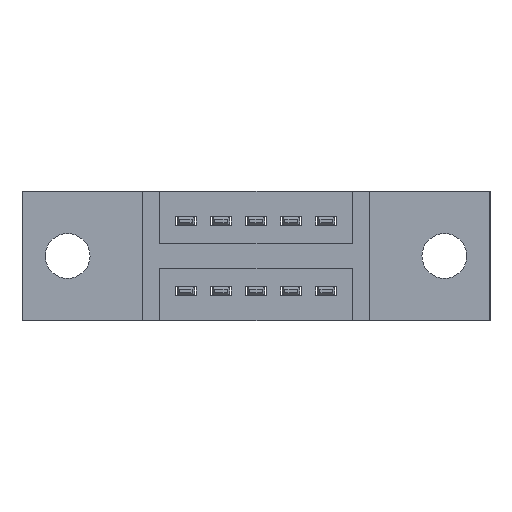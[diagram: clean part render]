
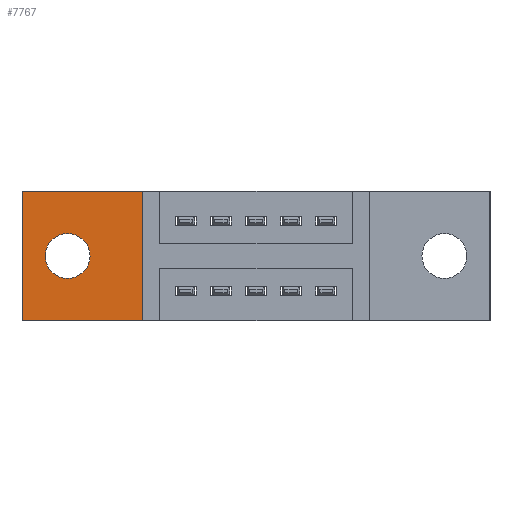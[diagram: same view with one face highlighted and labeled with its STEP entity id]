
A CAD part, front view. The second image highlights one B-rep face of the part: STEP entity #7767.
In plain terms, the highlighted planar face has unit normal (0, -1, 0).
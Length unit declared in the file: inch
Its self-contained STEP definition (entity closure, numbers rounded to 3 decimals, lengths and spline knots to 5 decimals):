
#136 = EDGE_LOOP ( 'NONE', ( #8341, #6078, #2822, #6022 ) ) ;
#354 = FACE_BOUND ( 'NONE', #4602, .T. ) ;
#615 = CARTESIAN_POINT ( 'NONE',  ( 0.3425, 0.17, 0. ) ) ;
#656 = VERTEX_POINT ( 'NONE', #5171 ) ;
#828 = DIRECTION ( 'NONE',  ( 0., 0., 1. ) ) ;
#831 = VERTEX_POINT ( 'NONE', #1865 ) ;
#839 = FACE_OUTER_BOUND ( 'NONE', #136, .T. ) ;
#1080 = CARTESIAN_POINT ( 'NONE',  ( 0., 0.17, -0.37 ) ) ;
#1251 = CARTESIAN_POINT ( 'NONE',  ( 0., 0.17, 0. ) ) ;
#1278 = DIRECTION ( 'NONE',  ( 0., 0., -1. ) ) ;
#1450 = CARTESIAN_POINT ( 'NONE',  ( 0.13, 0.17, -0.185 ) ) ;
#1543 = DIRECTION ( 'NONE',  ( 0., -1., 0. ) ) ;
#1711 = CARTESIAN_POINT ( 'NONE',  ( 0., 0.17, -0.37 ) ) ;
#1865 = CARTESIAN_POINT ( 'NONE',  ( 0.13, 0.17, -0.121 ) ) ;
#1981 = CIRCLE ( 'NONE', #6103, 0.064 ) ;
#2098 = VECTOR ( 'NONE', #1278, 39.37008 ) ;
#2188 = CARTESIAN_POINT ( 'NONE',  ( 0.13, 0.17, -0.249 ) ) ;
#2214 = VERTEX_POINT ( 'NONE', #5111 ) ;
#2232 = EDGE_CURVE ( 'NONE', #656, #2904, #4219, .T. ) ;
#2291 = VECTOR ( 'NONE', #828, 39.37008 ) ;
#2439 = LINE ( 'NONE', #1711, #7256 ) ;
#2822 = ORIENTED_EDGE ( 'NONE', *, *, #2232, .T. ) ;
#2904 = VERTEX_POINT ( 'NONE', #3269 ) ;
#3015 = CIRCLE ( 'NONE', #4152, 0.064 ) ;
#3106 = LINE ( 'NONE', #3818, #4953 ) ;
#3231 = DIRECTION ( 'NONE',  ( 0., -1., 0. ) ) ;
#3252 = VERTEX_POINT ( 'NONE', #2188 ) ;
#3269 = CARTESIAN_POINT ( 'NONE',  ( 0.3425, 0.17, 0. ) ) ;
#3818 = CARTESIAN_POINT ( 'NONE',  ( 0., 0.17, 0. ) ) ;
#4000 = LINE ( 'NONE', #1251, #2098 ) ;
#4152 = AXIS2_PLACEMENT_3D ( 'NONE', #1450, #1543, #6845 ) ;
#4219 = LINE ( 'NONE', #615, #2291 ) ;
#4441 = DIRECTION ( 'NONE',  ( -1., 0., 0. ) ) ;
#4602 = EDGE_LOOP ( 'NONE', ( #8755, #7608 ) ) ;
#4606 = EDGE_CURVE ( 'NONE', #3252, #831, #3015, .T. ) ;
#4778 = VERTEX_POINT ( 'NONE', #7077 ) ;
#4953 = VECTOR ( 'NONE', #4441, 39.37008 ) ;
#5095 = EDGE_CURVE ( 'NONE', #2904, #2214, #3106, .T. ) ;
#5111 = CARTESIAN_POINT ( 'NONE',  ( 0., 0.17, 0. ) ) ;
#5171 = CARTESIAN_POINT ( 'NONE',  ( 0.3425, 0.17, -0.37 ) ) ;
#5799 = DIRECTION ( 'NONE',  ( 0., 0., -1. ) ) ;
#5807 = CARTESIAN_POINT ( 'NONE',  ( 0.13, 0.17, -0.185 ) ) ;
#5833 = EDGE_CURVE ( 'NONE', #4778, #656, #2439, .T. ) ;
#6022 = ORIENTED_EDGE ( 'NONE', *, *, #5095, .T. ) ;
#6078 = ORIENTED_EDGE ( 'NONE', *, *, #5833, .T. ) ;
#6103 = AXIS2_PLACEMENT_3D ( 'NONE', #5807, #6502, #5799 ) ;
#6375 = EDGE_CURVE ( 'NONE', #831, #3252, #1981, .T. ) ;
#6502 = DIRECTION ( 'NONE',  ( 0., -1., 0. ) ) ;
#6845 = DIRECTION ( 'NONE',  ( 0., 0., -1. ) ) ;
#6870 = AXIS2_PLACEMENT_3D ( 'NONE', #1080, #3231, #7964 ) ;
#7077 = CARTESIAN_POINT ( 'NONE',  ( 0., 0.17, -0.37 ) ) ;
#7256 = VECTOR ( 'NONE', #8052, 39.37008 ) ;
#7311 = PLANE ( 'NONE',  #6870 ) ;
#7440 = EDGE_CURVE ( 'NONE', #2214, #4778, #4000, .T. ) ;
#7608 = ORIENTED_EDGE ( 'NONE', *, *, #4606, .F. ) ;
#7767 = ADVANCED_FACE ( 'NONE', ( #354, #839 ), #7311, .T. ) ;
#7964 = DIRECTION ( 'NONE',  ( 0., 0., -1. ) ) ;
#8052 = DIRECTION ( 'NONE',  ( 1., 0., 0. ) ) ;
#8341 = ORIENTED_EDGE ( 'NONE', *, *, #7440, .T. ) ;
#8755 = ORIENTED_EDGE ( 'NONE', *, *, #6375, .F. ) ;
